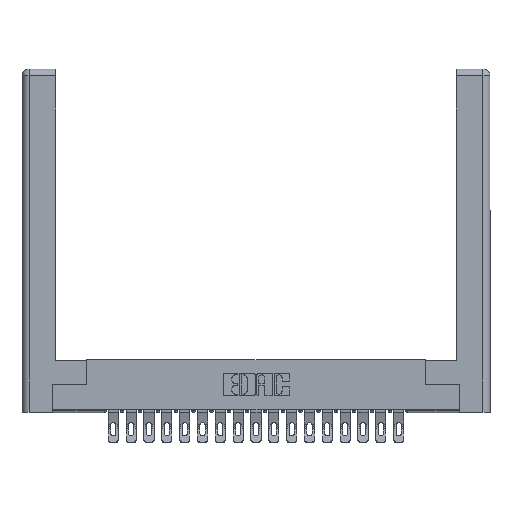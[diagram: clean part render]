
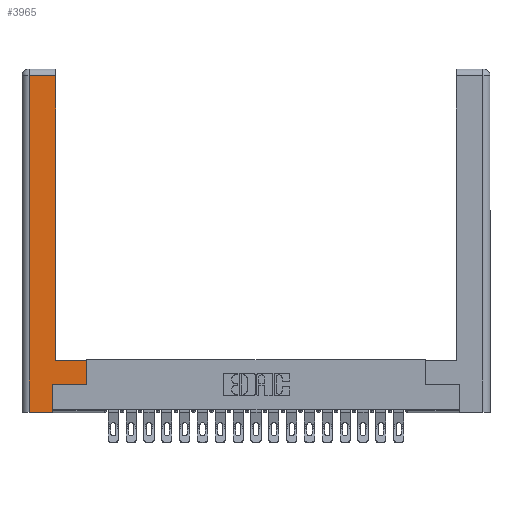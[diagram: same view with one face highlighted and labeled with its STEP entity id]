
A CAD part, top view. The second image highlights one B-rep face of the part: STEP entity #3965.
In plain terms, the highlighted planar face has unit normal (0, 0, 1).
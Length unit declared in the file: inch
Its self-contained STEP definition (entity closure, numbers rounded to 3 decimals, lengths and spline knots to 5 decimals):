
#188 = CARTESIAN_POINT ( 'NONE',  ( 0.0615, 0., 0. ) ) ;
#809 = CARTESIAN_POINT ( 'NONE',  ( 0.265, 0.245, 0. ) ) ;
#1185 = DIRECTION ( 'NONE',  ( 0., 0., -1. ) ) ;
#1249 = EDGE_CURVE ( 'NONE', #1411, #20550, #5323, .T. ) ;
#1319 = EDGE_CURVE ( 'NONE', #20550, #22555, #6019, .T. ) ;
#1411 = VERTEX_POINT ( 'NONE', #8203 ) ;
#1454 = CARTESIAN_POINT ( 'NONE',  ( 0.0615, 2.94, 0. ) ) ;
#1733 = CARTESIAN_POINT ( 'NONE',  ( 0.265, 0.245, 0. ) ) ;
#1825 = EDGE_CURVE ( 'NONE', #12634, #19538, #17902, .T. ) ;
#2325 = DIRECTION ( 'NONE',  ( 0., 1., 0. ) ) ;
#3965 = ADVANCED_FACE ( 'NONE', ( #4439 ), #8757, .F. ) ;
#4439 = FACE_OUTER_BOUND ( 'NONE', #14744, .T. ) ;
#5323 = LINE ( 'NONE', #1454, #22902 ) ;
#6013 = LINE ( 'NONE', #15916, #11664 ) ;
#6019 = LINE ( 'NONE', #18775, #17344 ) ;
#6689 = VERTEX_POINT ( 'NONE', #21282 ) ;
#7056 = EDGE_CURVE ( 'NONE', #23135, #18529, #7866, .T. ) ;
#7060 = ORIENTED_EDGE ( 'NONE', *, *, #23485, .T. ) ;
#7866 = LINE ( 'NONE', #12967, #22446 ) ;
#7881 = ORIENTED_EDGE ( 'NONE', *, *, #1825, .T. ) ;
#8203 = CARTESIAN_POINT ( 'NONE',  ( 0.295, 2.94, 0. ) ) ;
#8369 = EDGE_CURVE ( 'NONE', #19538, #1411, #18907, .T. ) ;
#8587 = VECTOR ( 'NONE', #20120, 39.37008 ) ;
#8757 = PLANE ( 'NONE',  #15188 ) ;
#10294 = EDGE_CURVE ( 'NONE', #22555, #6689, #6013, .T. ) ;
#10626 = CARTESIAN_POINT ( 'NONE',  ( 0.565, 0.45, 0. ) ) ;
#11664 = VECTOR ( 'NONE', #21625, 39.37008 ) ;
#11697 = ORIENTED_EDGE ( 'NONE', *, *, #10294, .T. ) ;
#11981 = CARTESIAN_POINT ( 'NONE',  ( 0.0615, 2.94, 0. ) ) ;
#12501 = CARTESIAN_POINT ( 'NONE',  ( 0.295, 0.45, 0. ) ) ;
#12634 = VERTEX_POINT ( 'NONE', #13669 ) ;
#12794 = VECTOR ( 'NONE', #17025, 39.37008 ) ;
#12967 = CARTESIAN_POINT ( 'NONE',  ( 0.565, 0.245, 0. ) ) ;
#13250 = DIRECTION ( 'NONE',  ( 0., -1., 0. ) ) ;
#13265 = ORIENTED_EDGE ( 'NONE', *, *, #8369, .T. ) ;
#13669 = CARTESIAN_POINT ( 'NONE',  ( 0.565, 0.45, 0. ) ) ;
#13862 = CARTESIAN_POINT ( 'NONE',  ( 0.295, 3., 0. ) ) ;
#14744 = EDGE_LOOP ( 'NONE', ( #13265, #17571, #20158, #11697, #16307, #23837, #7060, #7881 ) ) ;
#15188 = AXIS2_PLACEMENT_3D ( 'NONE', #18173, #1185, #22340 ) ;
#15916 = CARTESIAN_POINT ( 'NONE',  ( 0.265, 0., 0. ) ) ;
#16307 = ORIENTED_EDGE ( 'NONE', *, *, #20877, .T. ) ;
#16507 = DIRECTION ( 'NONE',  ( -1., 0., 0. ) ) ;
#17025 = DIRECTION ( 'NONE',  ( -1., 0., 0. ) ) ;
#17344 = VECTOR ( 'NONE', #13250, 39.37008 ) ;
#17571 = ORIENTED_EDGE ( 'NONE', *, *, #1249, .T. ) ;
#17652 = VECTOR ( 'NONE', #20746, 39.37008 ) ;
#17813 = LINE ( 'NONE', #10626, #8587 ) ;
#17902 = LINE ( 'NONE', #18858, #12794 ) ;
#18173 = CARTESIAN_POINT ( 'NONE',  ( 0., 0., 0. ) ) ;
#18529 = VERTEX_POINT ( 'NONE', #18540 ) ;
#18540 = CARTESIAN_POINT ( 'NONE',  ( 0.565, 0.245, 0. ) ) ;
#18775 = CARTESIAN_POINT ( 'NONE',  ( 0.0615, 0., 0. ) ) ;
#18858 = CARTESIAN_POINT ( 'NONE',  ( 0.295, 0.45, 0. ) ) ;
#18907 = LINE ( 'NONE', #13862, #23373 ) ;
#18917 = DIRECTION ( 'NONE',  ( 1., 0., 0. ) ) ;
#19538 = VERTEX_POINT ( 'NONE', #12501 ) ;
#20120 = DIRECTION ( 'NONE',  ( 0., 1., 0. ) ) ;
#20158 = ORIENTED_EDGE ( 'NONE', *, *, #1319, .T. ) ;
#20550 = VERTEX_POINT ( 'NONE', #11981 ) ;
#20746 = DIRECTION ( 'NONE',  ( 0., 1., 0. ) ) ;
#20877 = EDGE_CURVE ( 'NONE', #6689, #23135, #22736, .T. ) ;
#21282 = CARTESIAN_POINT ( 'NONE',  ( 0.265, 0., 0. ) ) ;
#21625 = DIRECTION ( 'NONE',  ( 1., 0., 0. ) ) ;
#22340 = DIRECTION ( 'NONE',  ( -1., 0., 0. ) ) ;
#22446 = VECTOR ( 'NONE', #18917, 39.37008 ) ;
#22555 = VERTEX_POINT ( 'NONE', #188 ) ;
#22736 = LINE ( 'NONE', #1733, #17652 ) ;
#22902 = VECTOR ( 'NONE', #16507, 39.37008 ) ;
#23135 = VERTEX_POINT ( 'NONE', #809 ) ;
#23373 = VECTOR ( 'NONE', #2325, 39.37008 ) ;
#23485 = EDGE_CURVE ( 'NONE', #18529, #12634, #17813, .T. ) ;
#23837 = ORIENTED_EDGE ( 'NONE', *, *, #7056, .T. ) ;
